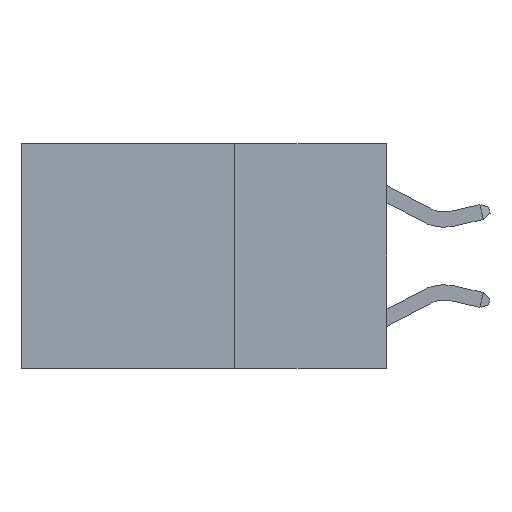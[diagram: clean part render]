
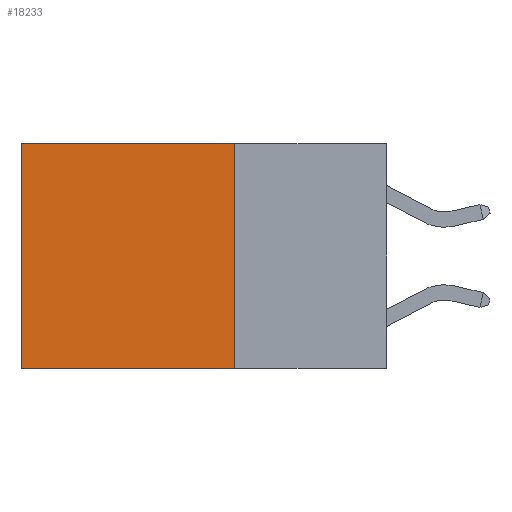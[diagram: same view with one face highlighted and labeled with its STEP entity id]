
A CAD part, left-side view. The second image highlights one B-rep face of the part: STEP entity #18233.
In plain terms, the highlighted planar face has unit normal (-1, 0, 0).
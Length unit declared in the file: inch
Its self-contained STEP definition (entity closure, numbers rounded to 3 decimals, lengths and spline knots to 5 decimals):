
#56 = DIRECTION ( 'NONE',  ( 1., 0., 0. ) ) ;
#232 = ORIENTED_EDGE ( 'NONE', *, *, #5608, .T. ) ;
#574 = VERTEX_POINT ( 'NONE', #8493 ) ;
#779 = ORIENTED_EDGE ( 'NONE', *, *, #13264, .F. ) ;
#2072 = VERTEX_POINT ( 'NONE', #18064 ) ;
#2468 = ORIENTED_EDGE ( 'NONE', *, *, #14093, .F. ) ;
#2539 = DIRECTION ( 'NONE',  ( 0., 1., 0. ) ) ;
#2902 = ORIENTED_EDGE ( 'NONE', *, *, #3462, .T. ) ;
#3462 = EDGE_CURVE ( 'NONE', #2072, #574, #18736, .T. ) ;
#3852 = DIRECTION ( 'NONE',  ( 0., 0., -1. ) ) ;
#4044 = CARTESIAN_POINT ( 'NONE',  ( 0.2625, 0.25, -0.37 ) ) ;
#5442 = EDGE_LOOP ( 'NONE', ( #232, #779, #2468, #2902 ) ) ;
#5608 = EDGE_CURVE ( 'NONE', #574, #15786, #13952, .T. ) ;
#5806 = CARTESIAN_POINT ( 'NONE',  ( 0.2625, 0.25, 0. ) ) ;
#6360 = CARTESIAN_POINT ( 'NONE',  ( 0.2625, 0.6, -0.37 ) ) ;
#6864 = FACE_OUTER_BOUND ( 'NONE', #5442, .T. ) ;
#7376 = DIRECTION ( 'NONE',  ( 0., 0., -1. ) ) ;
#8493 = CARTESIAN_POINT ( 'NONE',  ( 0.2625, 0.6, 0. ) ) ;
#8625 = AXIS2_PLACEMENT_3D ( 'NONE', #9089, #56, #10589 ) ;
#9089 = CARTESIAN_POINT ( 'NONE',  ( 0.2625, 0.25, 0. ) ) ;
#9999 = LINE ( 'NONE', #5806, #13554 ) ;
#10589 = DIRECTION ( 'NONE',  ( 0., 0., -1. ) ) ;
#12355 = CARTESIAN_POINT ( 'NONE',  ( 0.2625, 0.25, 0. ) ) ;
#12421 = DIRECTION ( 'NONE',  ( 0., 1., 0. ) ) ;
#12627 = LINE ( 'NONE', #4044, #16177 ) ;
#13264 = EDGE_CURVE ( 'NONE', #18219, #15786, #12627, .T. ) ;
#13475 = VECTOR ( 'NONE', #3852, 39.37008 ) ;
#13554 = VECTOR ( 'NONE', #7376, 39.37008 ) ;
#13586 = PLANE ( 'NONE',  #8625 ) ;
#13952 = LINE ( 'NONE', #14421, #13475 ) ;
#14093 = EDGE_CURVE ( 'NONE', #2072, #18219, #9999, .T. ) ;
#14421 = CARTESIAN_POINT ( 'NONE',  ( 0.2625, 0.6, 0. ) ) ;
#14766 = VECTOR ( 'NONE', #12421, 39.37008 ) ;
#15786 = VERTEX_POINT ( 'NONE', #6360 ) ;
#16177 = VECTOR ( 'NONE', #2539, 39.37008 ) ;
#17989 = CARTESIAN_POINT ( 'NONE',  ( 0.2625, 0.25, -0.37 ) ) ;
#18064 = CARTESIAN_POINT ( 'NONE',  ( 0.2625, 0.25, 0. ) ) ;
#18219 = VERTEX_POINT ( 'NONE', #17989 ) ;
#18233 = ADVANCED_FACE ( 'NONE', ( #6864 ), #13586, .F. ) ;
#18736 = LINE ( 'NONE', #12355, #14766 ) ;
